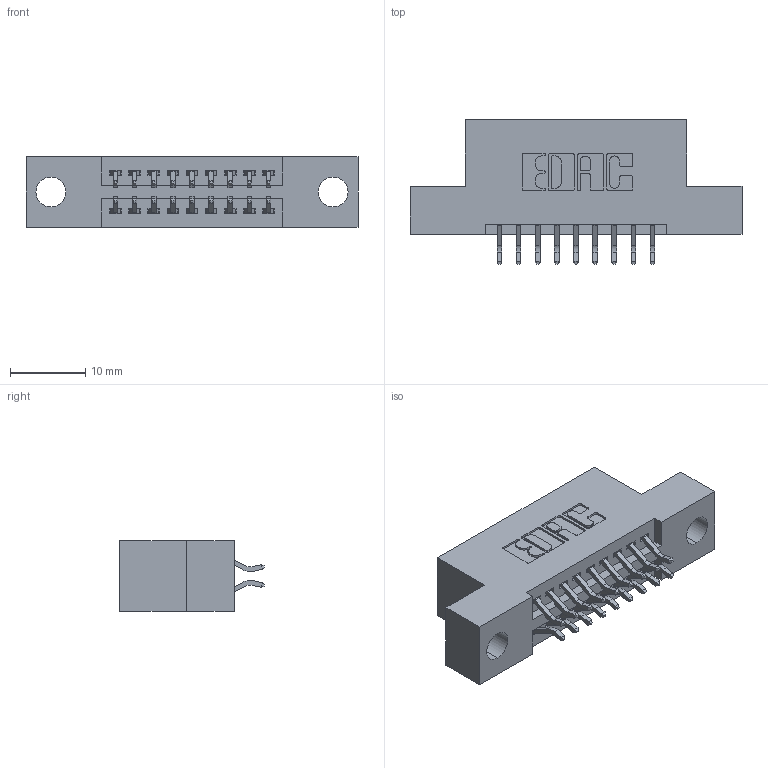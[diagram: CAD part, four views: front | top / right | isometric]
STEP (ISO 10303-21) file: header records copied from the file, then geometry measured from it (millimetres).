
FILE_DESCRIPTION (( 'STEP AP203' ), '1' );
FILE_NAME ('395-018-556-204.STEP', '2021-06-14T18:39:21', ( '' ), ( '' ), 'SwSTEP 2.0', 'SolidWorks 2020', '' );
FILE_SCHEMA (( 'CONFIG_CONTROL_DESIGN' ));
Length unit declared in the file: inch
Products named in the file (3): 395-018-556-204; 345 Part_Flush Mounting Lugs - 0.156 Dia-TI; 345-292-001_556 Tail
Assembly tree (19 placements, depth 2):
  395-018-556-204
    345 Part_Flush Mounting Lugs - 0.156 Dia-TI
    345-292-001_556 Tail  x18
Bounding box: 44.07 x 19.24 x 9.4 mm (x, y, z)
Volume: 3867.9 mm3; surface area: 4914.1 mm2
Topology: 19 solids, 19 shells, 1148 faces, 3383 edges, 2230 vertices
Faces by surface type: plane 760, cylinder 388
Entity records: 12143 total; most frequent: CARTESIAN_POINT 2086, ORIENTED_EDGE 2006, DIRECTION 1867, EDGE_CURVE 1003, VECTOR 827, LINE 827, VERTEX_POINT 666, AXIS2_PLACEMENT_3D 520
